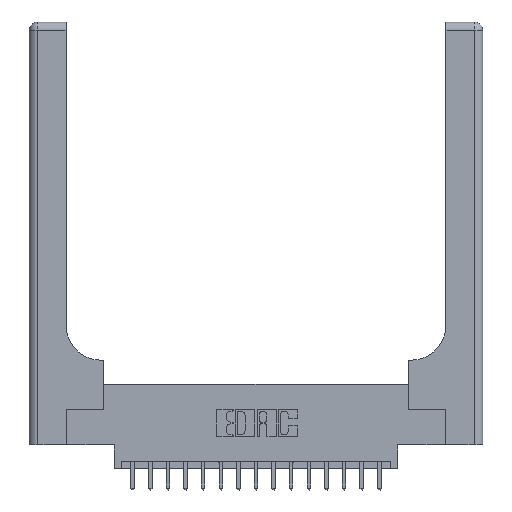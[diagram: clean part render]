
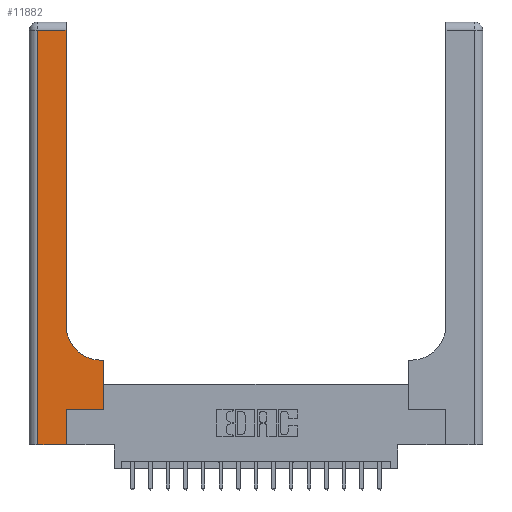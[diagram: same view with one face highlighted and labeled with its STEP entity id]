
A CAD part, top view. The second image highlights one B-rep face of the part: STEP entity #11882.
In plain terms, the highlighted planar face has unit normal (0, 0, 1).
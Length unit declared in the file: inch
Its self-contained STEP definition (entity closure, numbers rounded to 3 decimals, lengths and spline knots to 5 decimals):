
#975 = ORIENTED_EDGE ( 'NONE', *, *, #17550, .T. ) ;
#999 = VECTOR ( 'NONE', #7363, 39.37008 ) ;
#1023 = VECTOR ( 'NONE', #17104, 39.37008 ) ;
#1070 = LINE ( 'NONE', #15536, #16367 ) ;
#1202 = ORIENTED_EDGE ( 'NONE', *, *, #9049, .T. ) ;
#1246 = VECTOR ( 'NONE', #13431, 39.37008 ) ;
#1417 = CARTESIAN_POINT ( 'NONE',  ( 0.06, 0., 0.37 ) ) ;
#1557 = ORIENTED_EDGE ( 'NONE', *, *, #3907, .T. ) ;
#1938 = VERTEX_POINT ( 'NONE', #3478 ) ;
#2029 = DIRECTION ( 'NONE',  ( 0., 0., -1. ) ) ;
#2139 = LINE ( 'NONE', #8052, #11180 ) ;
#2225 = DIRECTION ( 'NONE',  ( 1., 0., 0. ) ) ;
#2474 = LINE ( 'NONE', #11597, #9699 ) ;
#3189 = CARTESIAN_POINT ( 'NONE',  ( 0.26, 0.6, 0.37 ) ) ;
#3478 = CARTESIAN_POINT ( 'NONE',  ( 0.51, 0.6, 0.37 ) ) ;
#3873 = PLANE ( 'NONE',  #16530 ) ;
#3907 = EDGE_CURVE ( 'NONE', #5553, #18689, #6679, .T. ) ;
#4243 = CARTESIAN_POINT ( 'NONE',  ( 0.265, 0.25, 0.37 ) ) ;
#4446 = LINE ( 'NONE', #13380, #10232 ) ;
#5553 = VERTEX_POINT ( 'NONE', #14033 ) ;
#5665 = DIRECTION ( 'NONE',  ( 1., 0., 0. ) ) ;
#5679 = DIRECTION ( 'NONE',  ( 0., 1., 0. ) ) ;
#5686 = VERTEX_POINT ( 'NONE', #1417 ) ;
#5767 = CARTESIAN_POINT ( 'NONE',  ( 0.51, 0.85, 0.37 ) ) ;
#6552 = CARTESIAN_POINT ( 'NONE',  ( 0.06, 2.94, 0.37 ) ) ;
#6679 = LINE ( 'NONE', #12601, #15173 ) ;
#6896 = EDGE_CURVE ( 'NONE', #5686, #11589, #10696, .T. ) ;
#7363 = DIRECTION ( 'NONE',  ( 0., 1., 0. ) ) ;
#7534 = DIRECTION ( 'NONE',  ( -1., 0., 0. ) ) ;
#7537 = EDGE_CURVE ( 'NONE', #10738, #5686, #2139, .T. ) ;
#7776 = EDGE_CURVE ( 'NONE', #18689, #10738, #4446, .T. ) ;
#8052 = CARTESIAN_POINT ( 'NONE',  ( 0.06, 3., 0.37 ) ) ;
#8599 = ORIENTED_EDGE ( 'NONE', *, *, #7776, .T. ) ;
#9049 = EDGE_CURVE ( 'NONE', #11589, #10849, #16408, .T. ) ;
#9100 = AXIS2_PLACEMENT_3D ( 'NONE', #5767, #15679, #5665 ) ;
#9627 = ORIENTED_EDGE ( 'NONE', *, *, #7537, .T. ) ;
#9699 = VECTOR ( 'NONE', #5679, 39.37008 ) ;
#9760 = ORIENTED_EDGE ( 'NONE', *, *, #11774, .T. ) ;
#9780 = CARTESIAN_POINT ( 'NONE',  ( 0., 3., 0.37 ) ) ;
#10232 = VECTOR ( 'NONE', #7534, 39.37008 ) ;
#10616 = CARTESIAN_POINT ( 'NONE',  ( 0.528, 0.25, 0.37 ) ) ;
#10696 = LINE ( 'NONE', #11769, #1246 ) ;
#10733 = ORIENTED_EDGE ( 'NONE', *, *, #12343, .T. ) ;
#10738 = VERTEX_POINT ( 'NONE', #6552 ) ;
#10849 = VERTEX_POINT ( 'NONE', #4243 ) ;
#11057 = FACE_OUTER_BOUND ( 'NONE', #19090, .T. ) ;
#11068 = DIRECTION ( 'NONE',  ( 0., -1., 0. ) ) ;
#11180 = VECTOR ( 'NONE', #11068, 39.37008 ) ;
#11589 = VERTEX_POINT ( 'NONE', #17315 ) ;
#11597 = CARTESIAN_POINT ( 'NONE',  ( 0.528, 0.25, 0.37 ) ) ;
#11769 = CARTESIAN_POINT ( 'NONE',  ( 0., 0., 0.37 ) ) ;
#11774 = EDGE_CURVE ( 'NONE', #13230, #1938, #16515, .T. ) ;
#11882 = ADVANCED_FACE ( 'NONE', ( #11057 ), #3873, .F. ) ;
#12343 = EDGE_CURVE ( 'NONE', #17042, #13230, #2474, .T. ) ;
#12601 = CARTESIAN_POINT ( 'NONE',  ( 0.26, 3., 0.37 ) ) ;
#13230 = VERTEX_POINT ( 'NONE', #14451 ) ;
#13380 = CARTESIAN_POINT ( 'NONE',  ( 0., 2.94, 0.37 ) ) ;
#13431 = DIRECTION ( 'NONE',  ( 1., 0., 0. ) ) ;
#13739 = CARTESIAN_POINT ( 'NONE',  ( 0.26, 2.94, 0.37 ) ) ;
#13880 = DIRECTION ( 'NONE',  ( -1., 0., 0. ) ) ;
#13940 = EDGE_CURVE ( 'NONE', #1938, #5553, #15324, .T. ) ;
#14033 = CARTESIAN_POINT ( 'NONE',  ( 0.26, 0.85, 0.37 ) ) ;
#14211 = ORIENTED_EDGE ( 'NONE', *, *, #13940, .T. ) ;
#14451 = CARTESIAN_POINT ( 'NONE',  ( 0.528, 0.6, 0.37 ) ) ;
#15173 = VECTOR ( 'NONE', #18560, 39.37008 ) ;
#15324 = CIRCLE ( 'NONE', #9100, 0.25 ) ;
#15536 = CARTESIAN_POINT ( 'NONE',  ( 0.265, 0.25, 0.37 ) ) ;
#15679 = DIRECTION ( 'NONE',  ( 0., 0., -1. ) ) ;
#16367 = VECTOR ( 'NONE', #2225, 39.37008 ) ;
#16408 = LINE ( 'NONE', #16505, #999 ) ;
#16505 = CARTESIAN_POINT ( 'NONE',  ( 0.265, 0., 0.37 ) ) ;
#16515 = LINE ( 'NONE', #3189, #1023 ) ;
#16530 = AXIS2_PLACEMENT_3D ( 'NONE', #9780, #2029, #13880 ) ;
#17042 = VERTEX_POINT ( 'NONE', #10616 ) ;
#17104 = DIRECTION ( 'NONE',  ( -1., 0., 0. ) ) ;
#17315 = CARTESIAN_POINT ( 'NONE',  ( 0.265, 0., 0.37 ) ) ;
#17550 = EDGE_CURVE ( 'NONE', #10849, #17042, #1070, .T. ) ;
#17629 = ORIENTED_EDGE ( 'NONE', *, *, #6896, .T. ) ;
#18560 = DIRECTION ( 'NONE',  ( 0., 1., 0. ) ) ;
#18689 = VERTEX_POINT ( 'NONE', #13739 ) ;
#19090 = EDGE_LOOP ( 'NONE', ( #1557, #8599, #9627, #17629, #1202, #975, #10733, #9760, #14211 ) ) ;
